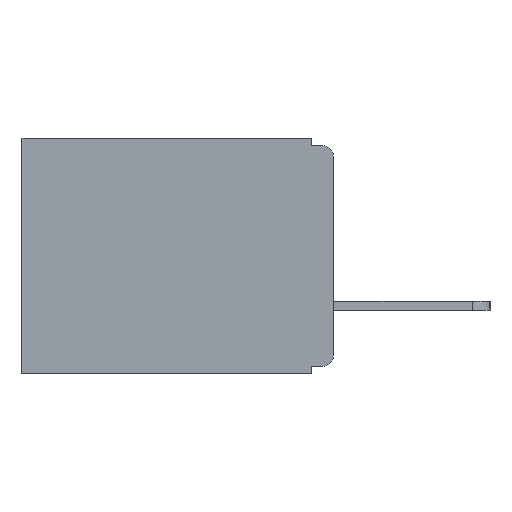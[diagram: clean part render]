
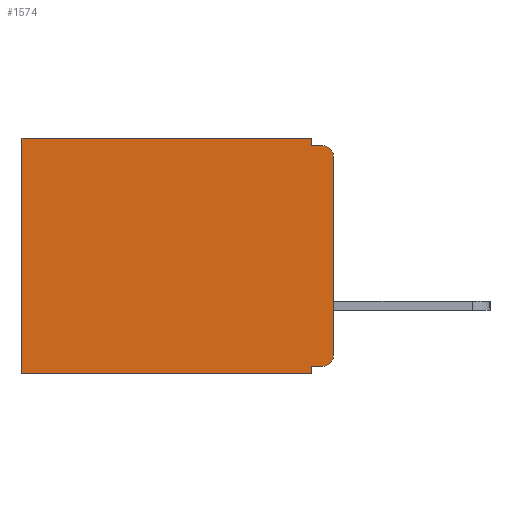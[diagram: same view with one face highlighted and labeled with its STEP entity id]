
A CAD part, left-side view. The second image highlights one B-rep face of the part: STEP entity #1574.
In plain terms, the highlighted planar face has unit normal (-1, 0, 0).
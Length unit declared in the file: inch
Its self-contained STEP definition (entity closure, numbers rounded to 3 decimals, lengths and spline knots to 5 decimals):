
#743 = ORIENTED_EDGE ( 'NONE', *, *, #13940, .F. ) ;
#916 = EDGE_CURVE ( 'NONE', #13347, #6230, #1040, .T. ) ;
#1040 = CIRCLE ( 'NONE', #14115, 0.015 ) ;
#1063 = EDGE_CURVE ( 'NONE', #16240, #5384, #18595, .T. ) ;
#1358 = ORIENTED_EDGE ( 'NONE', *, *, #5398, .T. ) ;
#1533 = DIRECTION ( 'NONE',  ( 0., 0., -1. ) ) ;
#1574 = ADVANCED_FACE ( 'NONE', ( #7249 ), #12837, .F. ) ;
#2073 = ORIENTED_EDGE ( 'NONE', *, *, #13664, .T. ) ;
#2081 = CARTESIAN_POINT ( 'NONE',  ( 0.3, 0., -0.025 ) ) ;
#2092 = EDGE_CURVE ( 'NONE', #13347, #11363, #16093, .T. ) ;
#2609 = ORIENTED_EDGE ( 'NONE', *, *, #14439, .F. ) ;
#2960 = ORIENTED_EDGE ( 'NONE', *, *, #1063, .F. ) ;
#3103 = VECTOR ( 'NONE', #6645, 39.37008 ) ;
#3139 = LINE ( 'NONE', #16183, #3103 ) ;
#3424 = ORIENTED_EDGE ( 'NONE', *, *, #8024, .F. ) ;
#3435 = CARTESIAN_POINT ( 'NONE',  ( 0.3, 0.031, -0.32 ) ) ;
#3691 = AXIS2_PLACEMENT_3D ( 'NONE', #15849, #15782, #15779 ) ;
#4100 = EDGE_LOOP ( 'NONE', ( #12832, #16482, #17837, #743, #1358, #2073, #2609, #2960, #3424, #5067 ) ) ;
#4192 = CARTESIAN_POINT ( 'NONE',  ( 0.3, 0., -0.33 ) ) ;
#4895 = VECTOR ( 'NONE', #5816, 39.37008 ) ;
#5035 = LINE ( 'NONE', #6239, #4895 ) ;
#5067 = ORIENTED_EDGE ( 'NONE', *, *, #11428, .T. ) ;
#5384 = VERTEX_POINT ( 'NONE', #8443 ) ;
#5398 = EDGE_CURVE ( 'NONE', #9570, #12020, #3139, .T. ) ;
#5816 = DIRECTION ( 'NONE',  ( 0., 1., 0. ) ) ;
#5930 = VERTEX_POINT ( 'NONE', #15321 ) ;
#6049 = VECTOR ( 'NONE', #16662, 39.37008 ) ;
#6208 = LINE ( 'NONE', #16151, #6049 ) ;
#6230 = VERTEX_POINT ( 'NONE', #17715 ) ;
#6239 = CARTESIAN_POINT ( 'NONE',  ( 0.3, 0., -0.33 ) ) ;
#6511 = CARTESIAN_POINT ( 'NONE',  ( 0.3, 0.015, -0.025 ) ) ;
#6586 = CARTESIAN_POINT ( 'NONE',  ( 0.3, 0.437, -0.33 ) ) ;
#6645 = DIRECTION ( 'NONE',  ( 0., 1., 0. ) ) ;
#6819 = VERTEX_POINT ( 'NONE', #6586 ) ;
#7249 = FACE_OUTER_BOUND ( 'NONE', #4100, .T. ) ;
#7486 = VERTEX_POINT ( 'NONE', #10002 ) ;
#7803 = VECTOR ( 'NONE', #9499, 39.37008 ) ;
#7894 = LINE ( 'NONE', #9654, #7803 ) ;
#8024 = EDGE_CURVE ( 'NONE', #5930, #16240, #8777, .T. ) ;
#8443 = CARTESIAN_POINT ( 'NONE',  ( 0.3, 0.031, -0.33 ) ) ;
#8641 = CIRCLE ( 'NONE', #3691, 0.015 ) ;
#8777 = LINE ( 'NONE', #18899, #12899 ) ;
#9499 = DIRECTION ( 'NONE',  ( 0., 0., -1. ) ) ;
#9561 = AXIS2_PLACEMENT_3D ( 'NONE', #17947, #12766, #15258 ) ;
#9570 = VERTEX_POINT ( 'NONE', #13091 ) ;
#9654 = CARTESIAN_POINT ( 'NONE',  ( 0.3, 0.031, 0. ) ) ;
#10002 = CARTESIAN_POINT ( 'NONE',  ( 0.3, 0.031, -0.01 ) ) ;
#10027 = VECTOR ( 'NONE', #17624, 39.37008 ) ;
#10049 = LINE ( 'NONE', #17602, #10027 ) ;
#10727 = DIRECTION ( 'NONE',  ( 0., 0., -1. ) ) ;
#11363 = VERTEX_POINT ( 'NONE', #18000 ) ;
#11428 = EDGE_CURVE ( 'NONE', #5930, #11363, #8641, .T. ) ;
#11455 = DIRECTION ( 'NONE',  ( 0., 0., -1. ) ) ;
#12020 = VERTEX_POINT ( 'NONE', #18350 ) ;
#12766 = DIRECTION ( 'NONE',  ( 1., 0., 0. ) ) ;
#12832 = ORIENTED_EDGE ( 'NONE', *, *, #2092, .F. ) ;
#12837 = PLANE ( 'NONE',  #9561 ) ;
#12899 = VECTOR ( 'NONE', #17928, 39.37008 ) ;
#13091 = CARTESIAN_POINT ( 'NONE',  ( 0.3, 0.031, 0. ) ) ;
#13347 = VERTEX_POINT ( 'NONE', #2081 ) ;
#13649 = CARTESIAN_POINT ( 'NONE',  ( 0.3, 0.031, -0.33 ) ) ;
#13664 = EDGE_CURVE ( 'NONE', #12020, #6819, #10049, .T. ) ;
#13940 = EDGE_CURVE ( 'NONE', #9570, #7486, #7894, .T. ) ;
#14115 = AXIS2_PLACEMENT_3D ( 'NONE', #6511, #15069, #1533 ) ;
#14273 = EDGE_CURVE ( 'NONE', #7486, #6230, #6208, .T. ) ;
#14439 = EDGE_CURVE ( 'NONE', #5384, #6819, #5035, .T. ) ;
#15069 = DIRECTION ( 'NONE',  ( -1., 0., 0. ) ) ;
#15258 = DIRECTION ( 'NONE',  ( 0., 0., -1. ) ) ;
#15321 = CARTESIAN_POINT ( 'NONE',  ( 0.3, 0.015, -0.32 ) ) ;
#15779 = DIRECTION ( 'NONE',  ( 0., 0., -1. ) ) ;
#15782 = DIRECTION ( 'NONE',  ( -1., 0., 0. ) ) ;
#15849 = CARTESIAN_POINT ( 'NONE',  ( 0.3, 0.015, -0.305 ) ) ;
#16015 = VECTOR ( 'NONE', #11455, 39.37008 ) ;
#16093 = LINE ( 'NONE', #4192, #16015 ) ;
#16151 = CARTESIAN_POINT ( 'NONE',  ( 0.3, 0., -0.01 ) ) ;
#16183 = CARTESIAN_POINT ( 'NONE',  ( 0.3, 0., 0. ) ) ;
#16240 = VERTEX_POINT ( 'NONE', #3435 ) ;
#16482 = ORIENTED_EDGE ( 'NONE', *, *, #916, .T. ) ;
#16662 = DIRECTION ( 'NONE',  ( 0., -1., 0. ) ) ;
#17602 = CARTESIAN_POINT ( 'NONE',  ( 0.3, 0.437, -0.33 ) ) ;
#17624 = DIRECTION ( 'NONE',  ( 0., 0., -1. ) ) ;
#17715 = CARTESIAN_POINT ( 'NONE',  ( 0.3, 0.015, -0.01 ) ) ;
#17837 = ORIENTED_EDGE ( 'NONE', *, *, #14273, .F. ) ;
#17928 = DIRECTION ( 'NONE',  ( 0., 1., 0. ) ) ;
#17947 = CARTESIAN_POINT ( 'NONE',  ( 0.3, 0., -0.33 ) ) ;
#18000 = CARTESIAN_POINT ( 'NONE',  ( 0.3, 0., -0.305 ) ) ;
#18262 = VECTOR ( 'NONE', #10727, 39.37008 ) ;
#18350 = CARTESIAN_POINT ( 'NONE',  ( 0.3, 0.437, 0. ) ) ;
#18595 = LINE ( 'NONE', #13649, #18262 ) ;
#18899 = CARTESIAN_POINT ( 'NONE',  ( 0.3, 0., -0.32 ) ) ;
